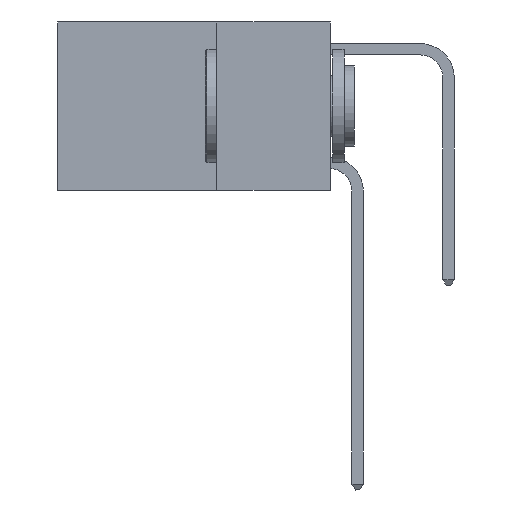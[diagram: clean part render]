
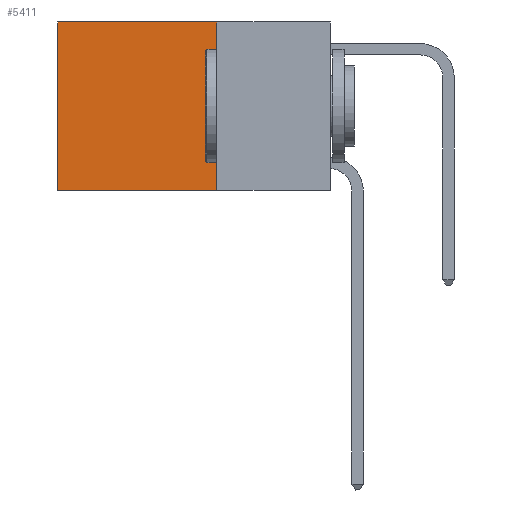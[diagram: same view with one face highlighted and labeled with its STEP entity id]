
A CAD part, left-side view. The second image highlights one B-rep face of the part: STEP entity #5411.
In plain terms, the highlighted planar face has unit normal (-1, 0, 0).
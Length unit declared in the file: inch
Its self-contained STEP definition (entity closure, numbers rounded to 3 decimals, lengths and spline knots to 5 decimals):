
#605 = VECTOR ( 'NONE', #2317, 39.37008 ) ;
#629 = LINE ( 'NONE', #11168, #13777 ) ;
#840 = EDGE_CURVE ( 'NONE', #1744, #10966, #629, .T. ) ;
#1744 = VERTEX_POINT ( 'NONE', #7098 ) ;
#2317 = DIRECTION ( 'NONE',  ( 0., 0., -1. ) ) ;
#2435 = CARTESIAN_POINT ( 'NONE',  ( 0.2625, 0.6, -0.37 ) ) ;
#2484 = VECTOR ( 'NONE', #10721, 39.37008 ) ;
#2518 = DIRECTION ( 'NONE',  ( 1., 0., 0. ) ) ;
#2523 = CARTESIAN_POINT ( 'NONE',  ( 0.2625, 0.6, 0. ) ) ;
#3031 = ORIENTED_EDGE ( 'NONE', *, *, #13481, .F. ) ;
#3188 = AXIS2_PLACEMENT_3D ( 'NONE', #9196, #2518, #15682 ) ;
#3903 = CARTESIAN_POINT ( 'NONE',  ( 0.2625, 0.25, 0. ) ) ;
#4912 = ORIENTED_EDGE ( 'NONE', *, *, #840, .F. ) ;
#5411 = ADVANCED_FACE ( 'NONE', ( #14684 ), #6385, .F. ) ;
#5800 = EDGE_CURVE ( 'NONE', #10848, #10966, #16161, .T. ) ;
#6075 = LINE ( 'NONE', #12697, #12675 ) ;
#6385 = PLANE ( 'NONE',  #3188 ) ;
#7098 = CARTESIAN_POINT ( 'NONE',  ( 0.2625, 0.25, -0.37 ) ) ;
#7240 = ORIENTED_EDGE ( 'NONE', *, *, #7863, .T. ) ;
#7863 = EDGE_CURVE ( 'NONE', #11283, #10848, #11936, .T. ) ;
#9196 = CARTESIAN_POINT ( 'NONE',  ( 0.2625, 0.25, 0. ) ) ;
#9965 = CARTESIAN_POINT ( 'NONE',  ( 0.2625, 0.25, 0. ) ) ;
#10721 = DIRECTION ( 'NONE',  ( 0., 1., 0. ) ) ;
#10848 = VERTEX_POINT ( 'NONE', #2523 ) ;
#10966 = VERTEX_POINT ( 'NONE', #2435 ) ;
#11168 = CARTESIAN_POINT ( 'NONE',  ( 0.2625, 0.25, -0.37 ) ) ;
#11283 = VERTEX_POINT ( 'NONE', #9965 ) ;
#11394 = DIRECTION ( 'NONE',  ( 0., 0., -1. ) ) ;
#11598 = CARTESIAN_POINT ( 'NONE',  ( 0.2625, 0.6, 0. ) ) ;
#11936 = LINE ( 'NONE', #3903, #2484 ) ;
#12675 = VECTOR ( 'NONE', #11394, 39.37008 ) ;
#12697 = CARTESIAN_POINT ( 'NONE',  ( 0.2625, 0.25, 0. ) ) ;
#13481 = EDGE_CURVE ( 'NONE', #11283, #1744, #6075, .T. ) ;
#13777 = VECTOR ( 'NONE', #16791, 39.37008 ) ;
#13782 = EDGE_LOOP ( 'NONE', ( #15565, #4912, #3031, #7240 ) ) ;
#14684 = FACE_OUTER_BOUND ( 'NONE', #13782, .T. ) ;
#15565 = ORIENTED_EDGE ( 'NONE', *, *, #5800, .T. ) ;
#15682 = DIRECTION ( 'NONE',  ( 0., 0., -1. ) ) ;
#16161 = LINE ( 'NONE', #11598, #605 ) ;
#16791 = DIRECTION ( 'NONE',  ( 0., 1., 0. ) ) ;
